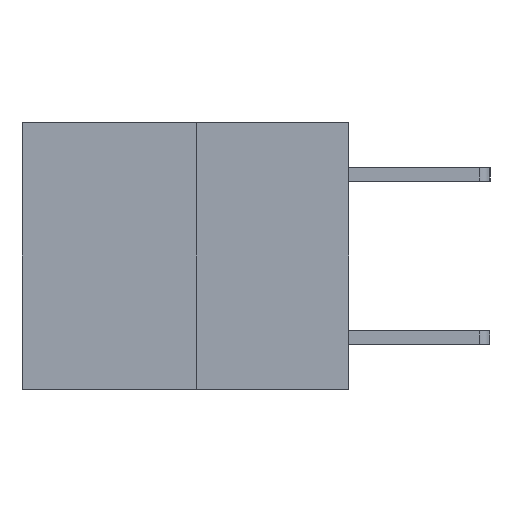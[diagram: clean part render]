
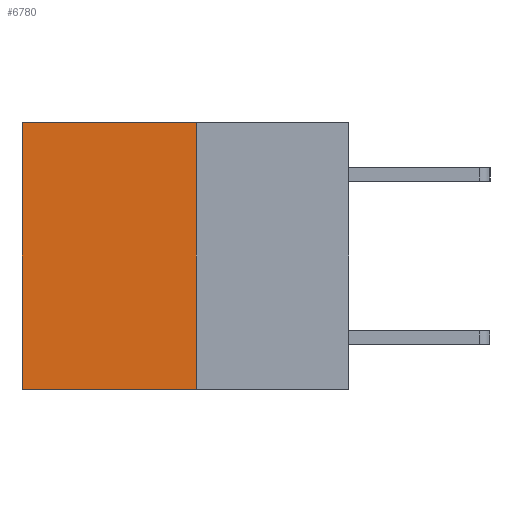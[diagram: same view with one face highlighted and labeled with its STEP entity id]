
A CAD part, left-side view. The second image highlights one B-rep face of the part: STEP entity #6780.
In plain terms, the highlighted planar face has unit normal (-1, 0, 0).
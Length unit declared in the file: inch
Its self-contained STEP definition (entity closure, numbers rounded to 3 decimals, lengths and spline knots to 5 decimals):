
#219 = VECTOR ( 'NONE', #6713, 39.37008 ) ;
#534 = VECTOR ( 'NONE', #4680, 39.37008 ) ;
#978 = LINE ( 'NONE', #3631, #4948 ) ;
#1012 = DIRECTION ( 'NONE',  ( 0., 1., 0. ) ) ;
#1152 = LINE ( 'NONE', #5357, #534 ) ;
#1345 = ORIENTED_EDGE ( 'NONE', *, *, #5431, .T. ) ;
#1793 = PLANE ( 'NONE',  #7129 ) ;
#1904 = EDGE_CURVE ( 'NONE', #8367, #6998, #5015, .T. ) ;
#2488 = FACE_OUTER_BOUND ( 'NONE', #4019, .T. ) ;
#2521 = CARTESIAN_POINT ( 'NONE',  ( 0.3165, 0.28, 0. ) ) ;
#3155 = CARTESIAN_POINT ( 'NONE',  ( 0.3165, 0.28, -0.49 ) ) ;
#3211 = ORIENTED_EDGE ( 'NONE', *, *, #3782, .T. ) ;
#3631 = CARTESIAN_POINT ( 'NONE',  ( 0.3165, 0.28, 0. ) ) ;
#3755 = DIRECTION ( 'NONE',  ( 1., 0., 0. ) ) ;
#3782 = EDGE_CURVE ( 'NONE', #8367, #7160, #978, .T. ) ;
#3939 = CARTESIAN_POINT ( 'NONE',  ( 0.3165, 0.6, 0. ) ) ;
#4019 = EDGE_LOOP ( 'NONE', ( #1345, #5910, #4138, #3211 ) ) ;
#4138 = ORIENTED_EDGE ( 'NONE', *, *, #1904, .F. ) ;
#4408 = LINE ( 'NONE', #8156, #5413 ) ;
#4680 = DIRECTION ( 'NONE',  ( 0., 1., 0. ) ) ;
#4948 = VECTOR ( 'NONE', #1012, 39.37008 ) ;
#5015 = LINE ( 'NONE', #5637, #219 ) ;
#5357 = CARTESIAN_POINT ( 'NONE',  ( 0.3165, 0.28, -0.49 ) ) ;
#5413 = VECTOR ( 'NONE', #6213, 39.37008 ) ;
#5431 = EDGE_CURVE ( 'NONE', #7160, #6669, #4408, .T. ) ;
#5556 = CARTESIAN_POINT ( 'NONE',  ( 0.3165, 0.6, -0.49 ) ) ;
#5637 = CARTESIAN_POINT ( 'NONE',  ( 0.3165, 0.28, -0.49 ) ) ;
#5910 = ORIENTED_EDGE ( 'NONE', *, *, #7740, .F. ) ;
#6213 = DIRECTION ( 'NONE',  ( 0., 0., -1. ) ) ;
#6669 = VERTEX_POINT ( 'NONE', #5556 ) ;
#6713 = DIRECTION ( 'NONE',  ( 0., 0., -1. ) ) ;
#6780 = ADVANCED_FACE ( 'NONE', ( #2488 ), #1793, .F. ) ;
#6998 = VERTEX_POINT ( 'NONE', #8312 ) ;
#7129 = AXIS2_PLACEMENT_3D ( 'NONE', #3155, #3755, #7718 ) ;
#7160 = VERTEX_POINT ( 'NONE', #3939 ) ;
#7718 = DIRECTION ( 'NONE',  ( 0., 0., -1. ) ) ;
#7740 = EDGE_CURVE ( 'NONE', #6998, #6669, #1152, .T. ) ;
#8156 = CARTESIAN_POINT ( 'NONE',  ( 0.3165, 0.6, -0.49 ) ) ;
#8312 = CARTESIAN_POINT ( 'NONE',  ( 0.3165, 0.28, -0.49 ) ) ;
#8367 = VERTEX_POINT ( 'NONE', #2521 ) ;
